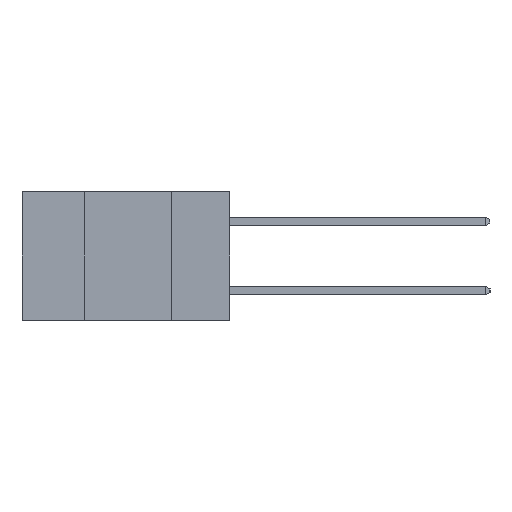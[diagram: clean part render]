
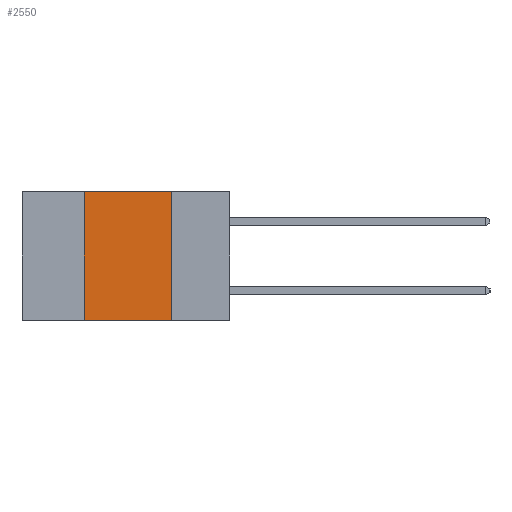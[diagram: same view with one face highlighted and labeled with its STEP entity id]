
A CAD part, left-side view. The second image highlights one B-rep face of the part: STEP entity #2550.
In plain terms, the highlighted planar face has unit normal (-1, 0, 0).
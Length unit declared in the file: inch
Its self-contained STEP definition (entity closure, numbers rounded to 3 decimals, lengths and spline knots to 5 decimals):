
#392 = LINE ( 'NONE', #6861, #1133 ) ;
#516 = CARTESIAN_POINT ( 'NONE',  ( 0., 0.6, 0. ) ) ;
#570 = PLANE ( 'NONE',  #1668 ) ;
#1133 = VECTOR ( 'NONE', #7350, 39.37008 ) ;
#1161 = DIRECTION ( 'NONE',  ( 1., 0., 0. ) ) ;
#1183 = VECTOR ( 'NONE', #7900, 39.37008 ) ;
#1656 = VERTEX_POINT ( 'NONE', #14211 ) ;
#1668 = AXIS2_PLACEMENT_3D ( 'NONE', #516, #1161, #3248 ) ;
#1950 = VERTEX_POINT ( 'NONE', #6603 ) ;
#2411 = VERTEX_POINT ( 'NONE', #7744 ) ;
#2550 = ADVANCED_FACE ( 'NONE', ( #11421 ), #570, .F. ) ;
#2596 = EDGE_LOOP ( 'NONE', ( #14380, #10516, #3612, #7131 ) ) ;
#2685 = VECTOR ( 'NONE', #11997, 39.37008 ) ;
#3248 = DIRECTION ( 'NONE',  ( 0., 0., -1. ) ) ;
#3563 = CARTESIAN_POINT ( 'NONE',  ( 0., 0.42, -0.37 ) ) ;
#3612 = ORIENTED_EDGE ( 'NONE', *, *, #4705, .F. ) ;
#3618 = DIRECTION ( 'NONE',  ( 0., 0., 1. ) ) ;
#4489 = LINE ( 'NONE', #3563, #10262 ) ;
#4705 = EDGE_CURVE ( 'NONE', #1950, #2411, #4489, .T. ) ;
#5500 = EDGE_CURVE ( 'NONE', #1950, #1656, #392, .T. ) ;
#6241 = VERTEX_POINT ( 'NONE', #9084 ) ;
#6603 = CARTESIAN_POINT ( 'NONE',  ( 0., 0.42, -0.37 ) ) ;
#6861 = CARTESIAN_POINT ( 'NONE',  ( 0., 0.6, -0.37 ) ) ;
#6941 = CARTESIAN_POINT ( 'NONE',  ( 0., 0.17, -0.37 ) ) ;
#7131 = ORIENTED_EDGE ( 'NONE', *, *, #5500, .T. ) ;
#7350 = DIRECTION ( 'NONE',  ( 0., -1., 0. ) ) ;
#7744 = CARTESIAN_POINT ( 'NONE',  ( 0., 0.42, 0. ) ) ;
#7900 = DIRECTION ( 'NONE',  ( 0., 0., -1. ) ) ;
#8375 = EDGE_CURVE ( 'NONE', #6241, #1656, #9884, .T. ) ;
#9084 = CARTESIAN_POINT ( 'NONE',  ( 0., 0.17, 0. ) ) ;
#9884 = LINE ( 'NONE', #6941, #1183 ) ;
#10262 = VECTOR ( 'NONE', #3618, 39.37008 ) ;
#10516 = ORIENTED_EDGE ( 'NONE', *, *, #12669, .F. ) ;
#11421 = FACE_OUTER_BOUND ( 'NONE', #2596, .T. ) ;
#11887 = CARTESIAN_POINT ( 'NONE',  ( 0., 0.6, 0. ) ) ;
#11988 = LINE ( 'NONE', #11887, #2685 ) ;
#11997 = DIRECTION ( 'NONE',  ( 0., -1., 0. ) ) ;
#12669 = EDGE_CURVE ( 'NONE', #2411, #6241, #11988, .T. ) ;
#14211 = CARTESIAN_POINT ( 'NONE',  ( 0., 0.17, -0.37 ) ) ;
#14380 = ORIENTED_EDGE ( 'NONE', *, *, #8375, .F. ) ;
